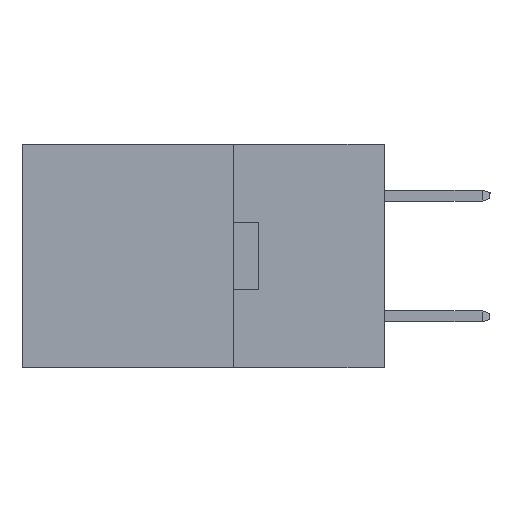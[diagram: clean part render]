
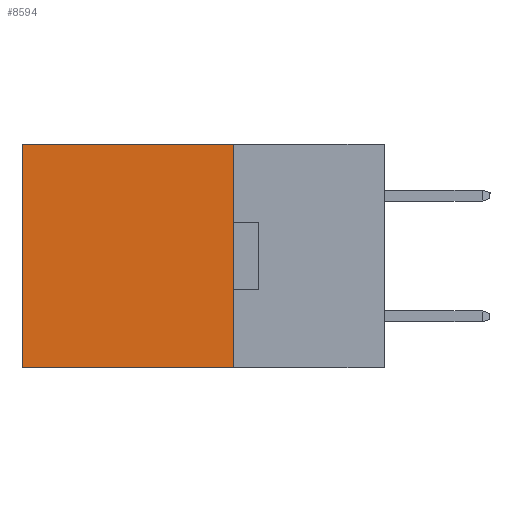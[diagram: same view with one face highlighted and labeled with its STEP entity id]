
A CAD part, left-side view. The second image highlights one B-rep face of the part: STEP entity #8594.
In plain terms, the highlighted planar face has unit normal (-1, 0, 0).
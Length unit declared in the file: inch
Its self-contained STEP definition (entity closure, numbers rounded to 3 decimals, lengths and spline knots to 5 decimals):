
#546 = VERTEX_POINT ( 'NONE', #5908 ) ;
#719 = CARTESIAN_POINT ( 'NONE',  ( 0.2615, 0.25, -0.37 ) ) ;
#1747 = VECTOR ( 'NONE', #18021, 39.37008 ) ;
#2109 = DIRECTION ( 'NONE',  ( 1., 0., 0. ) ) ;
#2150 = DIRECTION ( 'NONE',  ( 0., 1., 0. ) ) ;
#2874 = DIRECTION ( 'NONE',  ( 0., 1., 0. ) ) ;
#3156 = LINE ( 'NONE', #719, #13010 ) ;
#5908 = CARTESIAN_POINT ( 'NONE',  ( 0.2615, 0.25, -0.37 ) ) ;
#6495 = EDGE_CURVE ( 'NONE', #6717, #546, #3156, .T. ) ;
#6717 = VERTEX_POINT ( 'NONE', #15058 ) ;
#6880 = CARTESIAN_POINT ( 'NONE',  ( 0.2615, 0.6, 0. ) ) ;
#8002 = VECTOR ( 'NONE', #2150, 39.37008 ) ;
#8077 = CARTESIAN_POINT ( 'NONE',  ( 0.2615, 0.6, -0.37 ) ) ;
#8286 = VECTOR ( 'NONE', #2874, 39.37008 ) ;
#8594 = ADVANCED_FACE ( 'NONE', ( #17601 ), #26326, .F. ) ;
#8712 = EDGE_CURVE ( 'NONE', #24192, #19569, #9560, .T. ) ;
#8884 = ORIENTED_EDGE ( 'NONE', *, *, #8712, .T. ) ;
#9077 = AXIS2_PLACEMENT_3D ( 'NONE', #28187, #2109, #17312 ) ;
#9340 = LINE ( 'NONE', #22507, #8286 ) ;
#9560 = LINE ( 'NONE', #20165, #1747 ) ;
#13010 = VECTOR ( 'NONE', #18371, 39.37008 ) ;
#13964 = EDGE_CURVE ( 'NONE', #546, #19569, #9340, .T. ) ;
#15058 = CARTESIAN_POINT ( 'NONE',  ( 0.2615, 0.25, 0. ) ) ;
#16329 = ORIENTED_EDGE ( 'NONE', *, *, #20160, .T. ) ;
#17312 = DIRECTION ( 'NONE',  ( 0., 0., -1. ) ) ;
#17601 = FACE_OUTER_BOUND ( 'NONE', #20581, .T. ) ;
#17648 = LINE ( 'NONE', #24212, #8002 ) ;
#17700 = ORIENTED_EDGE ( 'NONE', *, *, #13964, .F. ) ;
#18021 = DIRECTION ( 'NONE',  ( 0., 0., -1. ) ) ;
#18371 = DIRECTION ( 'NONE',  ( 0., 0., -1. ) ) ;
#19569 = VERTEX_POINT ( 'NONE', #8077 ) ;
#20160 = EDGE_CURVE ( 'NONE', #6717, #24192, #17648, .T. ) ;
#20165 = CARTESIAN_POINT ( 'NONE',  ( 0.2615, 0.6, -0.37 ) ) ;
#20263 = ORIENTED_EDGE ( 'NONE', *, *, #6495, .F. ) ;
#20581 = EDGE_LOOP ( 'NONE', ( #8884, #17700, #20263, #16329 ) ) ;
#22507 = CARTESIAN_POINT ( 'NONE',  ( 0.2615, 0.25, -0.37 ) ) ;
#24192 = VERTEX_POINT ( 'NONE', #6880 ) ;
#24212 = CARTESIAN_POINT ( 'NONE',  ( 0.2615, 0.25, 0. ) ) ;
#26326 = PLANE ( 'NONE',  #9077 ) ;
#28187 = CARTESIAN_POINT ( 'NONE',  ( 0.2615, 0.25, -0.37 ) ) ;
